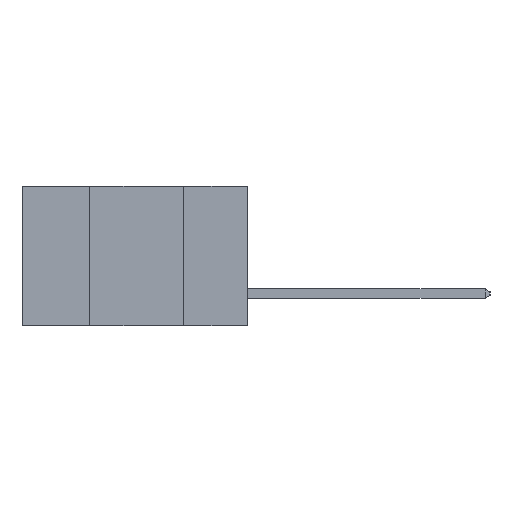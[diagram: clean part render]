
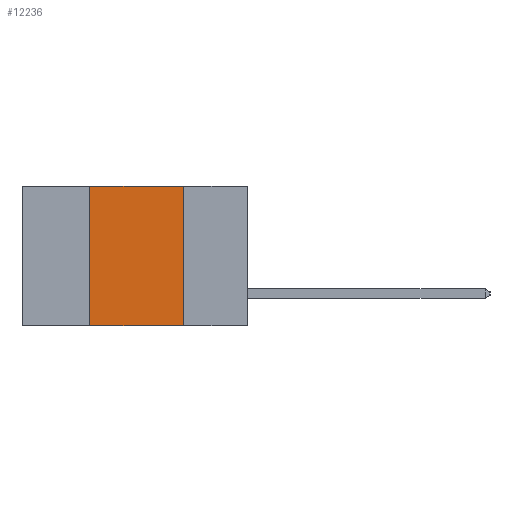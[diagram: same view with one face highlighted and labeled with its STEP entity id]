
A CAD part, left-side view. The second image highlights one B-rep face of the part: STEP entity #12236.
In plain terms, the highlighted planar face has unit normal (-1, 0, 0).
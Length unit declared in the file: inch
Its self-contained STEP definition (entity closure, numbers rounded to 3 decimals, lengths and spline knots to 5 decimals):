
#1473 = EDGE_CURVE ( 'NONE', #2745, #8165, #12182, .T. ) ;
#2745 = VERTEX_POINT ( 'NONE', #8838 ) ;
#3178 = VECTOR ( 'NONE', #5808, 39.37008 ) ;
#3364 = CARTESIAN_POINT ( 'NONE',  ( 0., 0.17, 0. ) ) ;
#3605 = FACE_OUTER_BOUND ( 'NONE', #8722, .T. ) ;
#4115 = PLANE ( 'NONE',  #13550 ) ;
#4257 = DIRECTION ( 'NONE',  ( 0., 0., 1. ) ) ;
#4276 = CARTESIAN_POINT ( 'NONE',  ( 0., 0.42, 0. ) ) ;
#4539 = LINE ( 'NONE', #4276, #13575 ) ;
#5001 = CARTESIAN_POINT ( 'NONE',  ( 0., 0.6, -0.37 ) ) ;
#5538 = EDGE_CURVE ( 'NONE', #12957, #6376, #11997, .T. ) ;
#5790 = CARTESIAN_POINT ( 'NONE',  ( 0., 0.17, -0.37 ) ) ;
#5808 = DIRECTION ( 'NONE',  ( 0., 0., -1. ) ) ;
#6376 = VERTEX_POINT ( 'NONE', #5790 ) ;
#6541 = DIRECTION ( 'NONE',  ( 0., 0., -1. ) ) ;
#7109 = EDGE_CURVE ( 'NONE', #12957, #2745, #4539, .T. ) ;
#7503 = ORIENTED_EDGE ( 'NONE', *, *, #7912, .F. ) ;
#7880 = ORIENTED_EDGE ( 'NONE', *, *, #1473, .F. ) ;
#7912 = EDGE_CURVE ( 'NONE', #8165, #6376, #12658, .T. ) ;
#8165 = VERTEX_POINT ( 'NONE', #12133 ) ;
#8722 = EDGE_LOOP ( 'NONE', ( #7503, #7880, #11029, #11377 ) ) ;
#8838 = CARTESIAN_POINT ( 'NONE',  ( 0., 0.42, 0. ) ) ;
#8887 = VECTOR ( 'NONE', #14232, 39.37008 ) ;
#10406 = CARTESIAN_POINT ( 'NONE',  ( 0., 0.42, -0.37 ) ) ;
#10458 = DIRECTION ( 'NONE',  ( 0., -1., 0. ) ) ;
#11029 = ORIENTED_EDGE ( 'NONE', *, *, #7109, .F. ) ;
#11377 = ORIENTED_EDGE ( 'NONE', *, *, #5538, .T. ) ;
#11830 = VECTOR ( 'NONE', #10458, 39.37008 ) ;
#11867 = CARTESIAN_POINT ( 'NONE',  ( 0., 0.6, 0. ) ) ;
#11997 = LINE ( 'NONE', #5001, #8887 ) ;
#12133 = CARTESIAN_POINT ( 'NONE',  ( 0., 0.17, 0. ) ) ;
#12182 = LINE ( 'NONE', #11867, #11830 ) ;
#12236 = ADVANCED_FACE ( 'NONE', ( #3605 ), #4115, .F. ) ;
#12418 = CARTESIAN_POINT ( 'NONE',  ( 0., 0.6, 0. ) ) ;
#12658 = LINE ( 'NONE', #3364, #3178 ) ;
#12957 = VERTEX_POINT ( 'NONE', #10406 ) ;
#13550 = AXIS2_PLACEMENT_3D ( 'NONE', #12418, #13570, #6541 ) ;
#13570 = DIRECTION ( 'NONE',  ( 1., 0., 0. ) ) ;
#13575 = VECTOR ( 'NONE', #4257, 39.37008 ) ;
#14232 = DIRECTION ( 'NONE',  ( 0., -1., 0. ) ) ;
